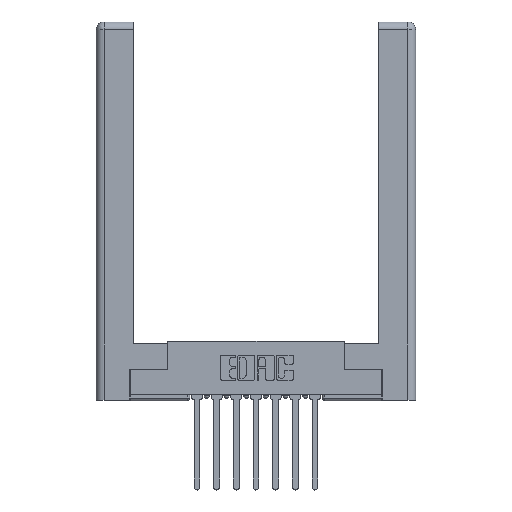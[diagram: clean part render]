
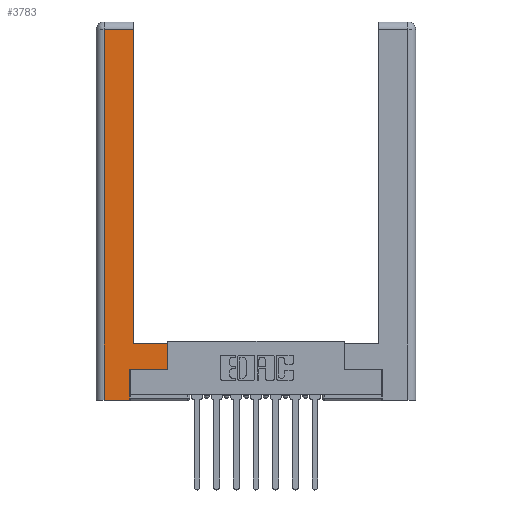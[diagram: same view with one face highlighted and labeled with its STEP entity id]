
A CAD part, top view. The second image highlights one B-rep face of the part: STEP entity #3783.
In plain terms, the highlighted planar face has unit normal (0, 0, 1).
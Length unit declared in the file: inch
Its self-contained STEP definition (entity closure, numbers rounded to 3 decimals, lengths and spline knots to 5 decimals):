
#110 = ORIENTED_EDGE ( 'NONE', *, *, #9701, .T. ) ;
#376 = VERTEX_POINT ( 'NONE', #12209 ) ;
#729 = LINE ( 'NONE', #11844, #10541 ) ;
#780 = EDGE_CURVE ( 'NONE', #2363, #12042, #9862, .T. ) ;
#1026 = CARTESIAN_POINT ( 'NONE',  ( 0.295, 0.45, 0. ) ) ;
#1220 = EDGE_CURVE ( 'NONE', #6774, #5110, #729, .T. ) ;
#1402 = ORIENTED_EDGE ( 'NONE', *, *, #10406, .T. ) ;
#1578 = VERTEX_POINT ( 'NONE', #8423 ) ;
#1631 = ORIENTED_EDGE ( 'NONE', *, *, #2615, .T. ) ;
#1665 = ORIENTED_EDGE ( 'NONE', *, *, #780, .T. ) ;
#1839 = CARTESIAN_POINT ( 'NONE',  ( 0.265, 0.245, 0. ) ) ;
#2124 = VECTOR ( 'NONE', #3959, 39.37008 ) ;
#2363 = VERTEX_POINT ( 'NONE', #9576 ) ;
#2458 = ORIENTED_EDGE ( 'NONE', *, *, #8968, .T. ) ;
#2610 = EDGE_LOOP ( 'NONE', ( #1631, #11230, #3861, #1402, #2458, #1665, #6791, #110 ) ) ;
#2615 = EDGE_CURVE ( 'NONE', #6104, #1578, #8963, .T. ) ;
#2648 = CARTESIAN_POINT ( 'NONE',  ( 0.265, 0., 0. ) ) ;
#2651 = VECTOR ( 'NONE', #11735, 39.37008 ) ;
#2813 = VERTEX_POINT ( 'NONE', #2648 ) ;
#3205 = CARTESIAN_POINT ( 'NONE',  ( 0.0615, 2.94, 0. ) ) ;
#3669 = CARTESIAN_POINT ( 'NONE',  ( 0.565, 0.245, 0. ) ) ;
#3751 = AXIS2_PLACEMENT_3D ( 'NONE', #9034, #10163, #11191 ) ;
#3783 = ADVANCED_FACE ( 'NONE', ( #9165 ), #12181, .F. ) ;
#3861 = ORIENTED_EDGE ( 'NONE', *, *, #1220, .T. ) ;
#3959 = DIRECTION ( 'NONE',  ( 0., 1., 0. ) ) ;
#4042 = VECTOR ( 'NONE', #7517, 39.37008 ) ;
#4089 = VECTOR ( 'NONE', #4799, 39.37008 ) ;
#4113 = CARTESIAN_POINT ( 'NONE',  ( 0.295, 3., 0. ) ) ;
#4212 = DIRECTION ( 'NONE',  ( 1., 0., 0. ) ) ;
#4799 = DIRECTION ( 'NONE',  ( 0., 1., 0. ) ) ;
#5110 = VERTEX_POINT ( 'NONE', #10738 ) ;
#5423 = CARTESIAN_POINT ( 'NONE',  ( 0.265, 0., 0. ) ) ;
#5652 = LINE ( 'NONE', #12665, #4089 ) ;
#5786 = DIRECTION ( 'NONE',  ( -1., 0., 0. ) ) ;
#6104 = VERTEX_POINT ( 'NONE', #1026 ) ;
#6753 = CARTESIAN_POINT ( 'NONE',  ( 0.565, 0.245, 0. ) ) ;
#6774 = VERTEX_POINT ( 'NONE', #3205 ) ;
#6791 = ORIENTED_EDGE ( 'NONE', *, *, #6923, .T. ) ;
#6895 = EDGE_CURVE ( 'NONE', #1578, #6774, #11791, .T. ) ;
#6923 = EDGE_CURVE ( 'NONE', #12042, #376, #5652, .T. ) ;
#7517 = DIRECTION ( 'NONE',  ( -1., 0., 0. ) ) ;
#8423 = CARTESIAN_POINT ( 'NONE',  ( 0.295, 2.94, 0. ) ) ;
#8963 = LINE ( 'NONE', #4113, #12450 ) ;
#8968 = EDGE_CURVE ( 'NONE', #2813, #2363, #9948, .T. ) ;
#9034 = CARTESIAN_POINT ( 'NONE',  ( 0., 0., 0. ) ) ;
#9165 = FACE_OUTER_BOUND ( 'NONE', #2610, .T. ) ;
#9576 = CARTESIAN_POINT ( 'NONE',  ( 0.265, 0.245, 0. ) ) ;
#9583 = VECTOR ( 'NONE', #4212, 39.37008 ) ;
#9647 = DIRECTION ( 'NONE',  ( 0., -1., 0. ) ) ;
#9701 = EDGE_CURVE ( 'NONE', #376, #6104, #9783, .T. ) ;
#9783 = LINE ( 'NONE', #11667, #4042 ) ;
#9862 = LINE ( 'NONE', #3669, #2651 ) ;
#9948 = LINE ( 'NONE', #1839, #2124 ) ;
#10161 = DIRECTION ( 'NONE',  ( 0., 1., 0. ) ) ;
#10163 = DIRECTION ( 'NONE',  ( 0., 0., -1. ) ) ;
#10406 = EDGE_CURVE ( 'NONE', #5110, #2813, #11626, .T. ) ;
#10541 = VECTOR ( 'NONE', #9647, 39.37008 ) ;
#10738 = CARTESIAN_POINT ( 'NONE',  ( 0.0615, 0., 0. ) ) ;
#11191 = DIRECTION ( 'NONE',  ( -1., 0., 0. ) ) ;
#11230 = ORIENTED_EDGE ( 'NONE', *, *, #6895, .T. ) ;
#11626 = LINE ( 'NONE', #5423, #9583 ) ;
#11667 = CARTESIAN_POINT ( 'NONE',  ( 0.295, 0.45, 0. ) ) ;
#11735 = DIRECTION ( 'NONE',  ( 1., 0., 0. ) ) ;
#11791 = LINE ( 'NONE', #12786, #12810 ) ;
#11844 = CARTESIAN_POINT ( 'NONE',  ( 0.0615, 0., 0. ) ) ;
#12042 = VERTEX_POINT ( 'NONE', #6753 ) ;
#12181 = PLANE ( 'NONE',  #3751 ) ;
#12209 = CARTESIAN_POINT ( 'NONE',  ( 0.565, 0.45, 0. ) ) ;
#12450 = VECTOR ( 'NONE', #10161, 39.37008 ) ;
#12665 = CARTESIAN_POINT ( 'NONE',  ( 0.565, 0.45, 0. ) ) ;
#12786 = CARTESIAN_POINT ( 'NONE',  ( 0.0615, 2.94, 0. ) ) ;
#12810 = VECTOR ( 'NONE', #5786, 39.37008 ) ;
